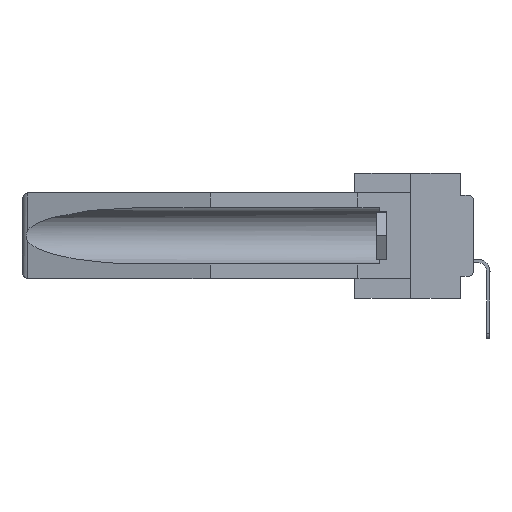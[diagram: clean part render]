
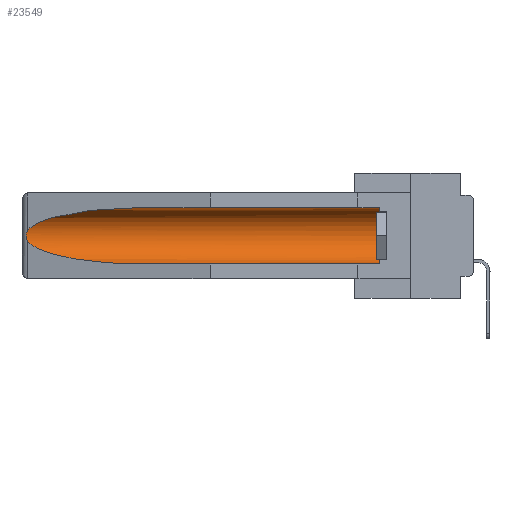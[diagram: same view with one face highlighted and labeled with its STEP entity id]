
A CAD part, left-side view. The second image highlights one B-rep face of the part: STEP entity #23549.
In plain terms, the highlighted cylindrical face has radius 2.857 mm (diameter 5.715 mm), a partial arc.
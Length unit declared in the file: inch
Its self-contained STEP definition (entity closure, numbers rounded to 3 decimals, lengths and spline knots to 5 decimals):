
#419 = CARTESIAN_POINT ( 'NONE',  ( 0.155, 0.126, -0.284 ) ) ;
#1381 = DIRECTION ( 'NONE',  ( 0., -1., 0. ) ) ;
#1415 = CARTESIAN_POINT ( 'NONE',  ( 0.26537, 1.52718, -0.19328 ) ) ;
#1951 = CARTESIAN_POINT ( 'NONE',  ( 0.155, -0.30754, -0.059 ) ) ;
#2520 = VECTOR ( 'NONE', #26883, 39.37008 ) ;
#3206 =( BOUNDED_CURVE ( )  B_SPLINE_CURVE ( 3, ( #28596, #9228, #28437, #4402 ),
 .UNSPECIFIED., .F., .F. ) 
 B_SPLINE_CURVE_WITH_KNOTS ( ( 4, 4 ),
 ( 4.71239, 6.08839 ),
 .UNSPECIFIED. ) 
 CURVE ( )  GEOMETRIC_REPRESENTATION_ITEM ( )  RATIONAL_B_SPLINE_CURVE ( ( 1., 0.848, 0.848, 1. ) ) 
 REPRESENTATION_ITEM ( '' )  );
#3207 = CARTESIAN_POINT ( 'NONE',  ( 0.155, -0.30754, -0.1715 ) ) ;
#4357 = ORIENTED_EDGE ( 'NONE', *, *, #18786, .T. ) ;
#4402 = CARTESIAN_POINT ( 'NONE',  ( 0.26537, 1.52718, -0.14972 ) ) ;
#4621 = VECTOR ( 'NONE', #21201, 39.37008 ) ;
#5013 = CARTESIAN_POINT ( 'NONE',  ( 0.26597, 1.52961, -0.15275 ) ) ;
#5203 = CARTESIAN_POINT ( 'NONE',  ( 0.2675, 1.53308, -0.17534 ) ) ;
#5816 = CARTESIAN_POINT ( 'NONE',  ( 0.155, 1.07973, -0.059 ) ) ;
#6341 = CARTESIAN_POINT ( 'NONE',  ( 0.155, 0.126, -0.1715 ) ) ;
#6382 = CARTESIAN_POINT ( 'NONE',  ( 0.25451, 1.48313, -0.24835 ) ) ;
#6913 = EDGE_CURVE ( 'NONE', #28336, #17279, #15100, .T. ) ;
#7838 = LINE ( 'NONE', #18432, #2520 ) ;
#8019 = DIRECTION ( 'NONE',  ( 0., 1., 0. ) ) ;
#8343 = FACE_OUTER_BOUND ( 'NONE', #33656, .T. ) ;
#8372 = CARTESIAN_POINT ( 'NONE',  ( 0.26654, 1.53092, -0.15636 ) ) ;
#8517 = CARTESIAN_POINT ( 'NONE',  ( 0.155, 0.126, -0.059 ) ) ;
#9228 = CARTESIAN_POINT ( 'NONE',  ( 0.21114, 1.30732, -0.059 ) ) ;
#9455 = ORIENTED_EDGE ( 'NONE', *, *, #25777, .T. ) ;
#11265 = EDGE_CURVE ( 'NONE', #26986, #20108, #7838, .T. ) ;
#11413 = CARTESIAN_POINT ( 'NONE',  ( 0.26537, 1.52718, -0.14972 ) ) ;
#12982 = VERTEX_POINT ( 'NONE', #5816 ) ;
#13328 = CARTESIAN_POINT ( 'NONE',  ( 0.26655, 1.53094, -0.18657 ) ) ;
#14660 = CARTESIAN_POINT ( 'NONE',  ( 0.21114, 1.30732, -0.284 ) ) ;
#15100 = B_SPLINE_CURVE_WITH_KNOTS ( 'NONE', 3,
 ( #21105, #5013, #8372, #26371, #16153, #5203, #26898, #13328, #21262, #32033 ),
 .UNSPECIFIED., .F., .F.,
 ( 4, 2, 2, 2, 4 ),
 ( 0., 0.00029, 0.00058, 0.00087, 0.00117 ),
 .UNSPECIFIED. ) ;
#15196 = ORIENTED_EDGE ( 'NONE', *, *, #6913, .T. ) ;
#16153 = CARTESIAN_POINT ( 'NONE',  ( 0.2675, 1.53308, -0.16763 ) ) ;
#17279 = VERTEX_POINT ( 'NONE', #24032 ) ;
#18432 = CARTESIAN_POINT ( 'NONE',  ( 0.155, -0.30754, -0.284 ) ) ;
#18786 = EDGE_CURVE ( 'NONE', #17279, #20108, #21476, .T. ) ;
#19302 = CYLINDRICAL_SURFACE ( 'NONE', #28953, 0.1125 ) ;
#20108 = VERTEX_POINT ( 'NONE', #30088 ) ;
#20320 = AXIS2_PLACEMENT_3D ( 'NONE', #6341, #1381, #30698 ) ;
#20630 = VERTEX_POINT ( 'NONE', #8517 ) ;
#21105 = CARTESIAN_POINT ( 'NONE',  ( 0.26537, 1.52718, -0.14972 ) ) ;
#21171 = EDGE_CURVE ( 'NONE', #26986, #20630, #31625, .T. ) ;
#21201 = DIRECTION ( 'NONE',  ( 0., 1., 0. ) ) ;
#21262 = CARTESIAN_POINT ( 'NONE',  ( 0.26597, 1.5296, -0.19026 ) ) ;
#21476 =( BOUNDED_CURVE ( )  B_SPLINE_CURVE ( 3, ( #1415, #6382, #14660, #30889 ),
 .UNSPECIFIED., .F., .F. ) 
 B_SPLINE_CURVE_WITH_KNOTS ( ( 4, 4 ),
 ( 0.1948, 1.5708 ),
 .UNSPECIFIED. ) 
 CURVE ( )  GEOMETRIC_REPRESENTATION_ITEM ( )  RATIONAL_B_SPLINE_CURVE ( ( 1., 0.848, 0.848, 1. ) ) 
 REPRESENTATION_ITEM ( '' )  );
#22201 = EDGE_CURVE ( 'NONE', #20630, #12982, #32141, .T. ) ;
#23549 = ADVANCED_FACE ( 'NONE', ( #8343 ), #19302, .F. ) ;
#24032 = CARTESIAN_POINT ( 'NONE',  ( 0.26537, 1.52718, -0.19328 ) ) ;
#25312 = ORIENTED_EDGE ( 'NONE', *, *, #11265, .F. ) ;
#25777 = EDGE_CURVE ( 'NONE', #12982, #28336, #3206, .T. ) ;
#26371 = CARTESIAN_POINT ( 'NONE',  ( 0.2673, 1.5327, -0.16383 ) ) ;
#26883 = DIRECTION ( 'NONE',  ( 0., 1., 0. ) ) ;
#26898 = CARTESIAN_POINT ( 'NONE',  ( 0.2673, 1.53269, -0.17917 ) ) ;
#26986 = VERTEX_POINT ( 'NONE', #419 ) ;
#28336 = VERTEX_POINT ( 'NONE', #11413 ) ;
#28437 = CARTESIAN_POINT ( 'NONE',  ( 0.25451, 1.48313, -0.09465 ) ) ;
#28596 = CARTESIAN_POINT ( 'NONE',  ( 0.155, 1.07973, -0.059 ) ) ;
#28953 = AXIS2_PLACEMENT_3D ( 'NONE', #3207, #8019, #29875 ) ;
#29647 = ORIENTED_EDGE ( 'NONE', *, *, #22201, .T. ) ;
#29875 = DIRECTION ( 'NONE',  ( 0., 0., 1. ) ) ;
#30088 = CARTESIAN_POINT ( 'NONE',  ( 0.155, 1.07973, -0.284 ) ) ;
#30698 = DIRECTION ( 'NONE',  ( 0., 0., 1. ) ) ;
#30889 = CARTESIAN_POINT ( 'NONE',  ( 0.155, 1.07973, -0.284 ) ) ;
#30934 = ORIENTED_EDGE ( 'NONE', *, *, #21171, .T. ) ;
#31625 = CIRCLE ( 'NONE', #20320, 0.1125 ) ;
#32033 = CARTESIAN_POINT ( 'NONE',  ( 0.26537, 1.52718, -0.19328 ) ) ;
#32141 = LINE ( 'NONE', #1951, #4621 ) ;
#33656 = EDGE_LOOP ( 'NONE', ( #9455, #15196, #4357, #25312, #30934, #29647 ) ) ;
